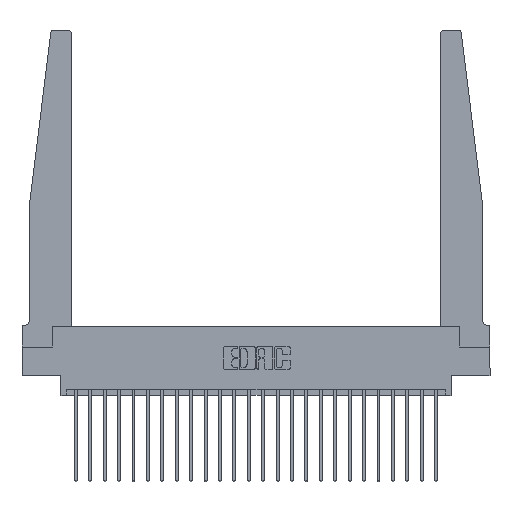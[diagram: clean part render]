
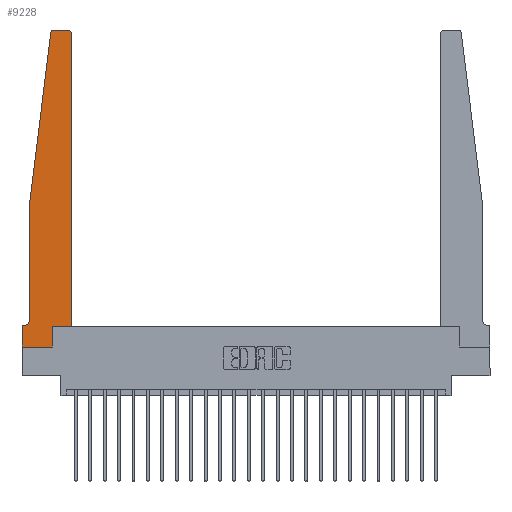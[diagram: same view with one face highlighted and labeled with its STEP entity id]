
A CAD part, top view. The second image highlights one B-rep face of the part: STEP entity #9228.
In plain terms, the highlighted planar face has unit normal (0, 0, 1).
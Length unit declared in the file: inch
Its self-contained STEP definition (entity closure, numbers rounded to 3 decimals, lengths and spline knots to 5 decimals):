
#32 = EDGE_LOOP ( 'NONE', ( #1885, #21672, #7446, #8039, #13606, #23380, #9219, #429, #5406, #1018, #11001, #21397 ) ) ;
#429 = ORIENTED_EDGE ( 'NONE', *, *, #17826, .T. ) ;
#541 = CARTESIAN_POINT ( 'NONE',  ( 0.425, 0.18, 0.37 ) ) ;
#664 = LINE ( 'NONE', #5617, #23602 ) ;
#988 = CARTESIAN_POINT ( 'NONE',  ( 0.065, 0.2375, 0.37 ) ) ;
#1018 = ORIENTED_EDGE ( 'NONE', *, *, #8306, .T. ) ;
#1086 = LINE ( 'NONE', #17839, #20286 ) ;
#1133 = VECTOR ( 'NONE', #13328, 39.37008 ) ;
#1623 = CARTESIAN_POINT ( 'NONE',  ( 0.015, 0.2375, 0.37 ) ) ;
#1766 = CARTESIAN_POINT ( 'NONE',  ( 0.395, 2.72, 0.37 ) ) ;
#1885 = ORIENTED_EDGE ( 'NONE', *, *, #13297, .T. ) ;
#2286 = VECTOR ( 'NONE', #2772, 39.37008 ) ;
#2309 = LINE ( 'NONE', #15104, #1133 ) ;
#2438 = CIRCLE ( 'NONE', #17186, 0.05 ) ;
#2493 = CARTESIAN_POINT ( 'NONE',  ( 0.27653, 2.72, 0.37 ) ) ;
#2772 = DIRECTION ( 'NONE',  ( -1., 0., 0. ) ) ;
#2849 = DIRECTION ( 'NONE',  ( 0., -1., 0. ) ) ;
#3151 = CIRCLE ( 'NONE', #17919, 0.03 ) ;
#3530 = DIRECTION ( 'NONE',  ( -1., 0., 0. ) ) ;
#3667 = LINE ( 'NONE', #15150, #22817 ) ;
#3668 = DIRECTION ( 'NONE',  ( 1., 0., 0. ) ) ;
#4376 = DIRECTION ( 'NONE',  ( 1., 0., 0. ) ) ;
#4550 = DIRECTION ( 'NONE',  ( 1., 0., 0. ) ) ;
#4592 = DIRECTION ( 'NONE',  ( -1., 0., 0. ) ) ;
#4704 = CARTESIAN_POINT ( 'NONE',  ( 0., 0.1875, 0.37 ) ) ;
#4827 = CIRCLE ( 'NONE', #8594, 0.03 ) ;
#5361 = EDGE_CURVE ( 'NONE', #18653, #9847, #21403, .T. ) ;
#5406 = ORIENTED_EDGE ( 'NONE', *, *, #10839, .T. ) ;
#5617 = CARTESIAN_POINT ( 'NONE',  ( 0.425, 0.18, 0.37 ) ) ;
#5650 = CARTESIAN_POINT ( 'NONE',  ( 0.395, 2.75, 0.37 ) ) ;
#6002 = VECTOR ( 'NONE', #2849, 39.37008 ) ;
#6142 = VERTEX_POINT ( 'NONE', #18360 ) ;
#6535 = CARTESIAN_POINT ( 'NONE',  ( 0.065, 1.25, 0.37 ) ) ;
#6582 = DIRECTION ( 'NONE',  ( 0., 0., 1. ) ) ;
#7446 = ORIENTED_EDGE ( 'NONE', *, *, #14765, .T. ) ;
#7843 = LINE ( 'NONE', #12108, #2286 ) ;
#7942 = AXIS2_PLACEMENT_3D ( 'NONE', #4704, #6582, #19578 ) ;
#7964 = VECTOR ( 'NONE', #4550, 39.37008 ) ;
#8039 = ORIENTED_EDGE ( 'NONE', *, *, #5361, .T. ) ;
#8271 = CARTESIAN_POINT ( 'NONE',  ( 0.2605, 0., 0.37 ) ) ;
#8306 = EDGE_CURVE ( 'NONE', #14485, #17707, #2309, .T. ) ;
#8594 = AXIS2_PLACEMENT_3D ( 'NONE', #1766, #14836, #3668 ) ;
#9219 = ORIENTED_EDGE ( 'NONE', *, *, #15057, .T. ) ;
#9228 = ADVANCED_FACE ( 'NONE', ( #13394 ), #21348, .T. ) ;
#9348 = CARTESIAN_POINT ( 'NONE',  ( 0., 0., 0.37 ) ) ;
#9451 = VECTOR ( 'NONE', #4592, 39.37008 ) ;
#9847 = VERTEX_POINT ( 'NONE', #988 ) ;
#10765 = EDGE_CURVE ( 'NONE', #13811, #11398, #4827, .T. ) ;
#10839 = EDGE_CURVE ( 'NONE', #13287, #14485, #3667, .T. ) ;
#11001 = ORIENTED_EDGE ( 'NONE', *, *, #17537, .T. ) ;
#11361 = VECTOR ( 'NONE', #17218, 39.37008 ) ;
#11398 = VERTEX_POINT ( 'NONE', #5650 ) ;
#11630 = CARTESIAN_POINT ( 'NONE',  ( 0.065, 1.25, 0.37 ) ) ;
#11886 = EDGE_CURVE ( 'NONE', #9847, #21925, #2438, .T. ) ;
#12012 = CARTESIAN_POINT ( 'NONE',  ( 0., 0., 0.37 ) ) ;
#12053 = CARTESIAN_POINT ( 'NONE',  ( 0.25, 2.75, 0.37 ) ) ;
#12108 = CARTESIAN_POINT ( 'NONE',  ( 0.065, 0.1875, 0.37 ) ) ;
#13287 = VERTEX_POINT ( 'NONE', #8271 ) ;
#13297 = EDGE_CURVE ( 'NONE', #11398, #17011, #14403, .T. ) ;
#13328 = DIRECTION ( 'NONE',  ( 1., 0., 0. ) ) ;
#13394 = FACE_OUTER_BOUND ( 'NONE', #32, .T. ) ;
#13606 = ORIENTED_EDGE ( 'NONE', *, *, #11886, .T. ) ;
#13811 = VERTEX_POINT ( 'NONE', #21604 ) ;
#14403 = LINE ( 'NONE', #12053, #9451 ) ;
#14485 = VERTEX_POINT ( 'NONE', #19788 ) ;
#14696 = DIRECTION ( 'NONE',  ( 0., 0., -1. ) ) ;
#14765 = EDGE_CURVE ( 'NONE', #6142, #18653, #16291, .T. ) ;
#14836 = DIRECTION ( 'NONE',  ( 0., 0., 1. ) ) ;
#14935 = DIRECTION ( 'NONE',  ( 0., 1., 0. ) ) ;
#15057 = EDGE_CURVE ( 'NONE', #23417, #22206, #1086, .T. ) ;
#15104 = CARTESIAN_POINT ( 'NONE',  ( 0.425, 0.18, 0.37 ) ) ;
#15150 = CARTESIAN_POINT ( 'NONE',  ( 0.2605, 0.18, 0.37 ) ) ;
#15564 = DIRECTION ( 'NONE',  ( 0., 0., 1. ) ) ;
#16291 = LINE ( 'NONE', #11630, #11361 ) ;
#17011 = VERTEX_POINT ( 'NONE', #19065 ) ;
#17015 = DIRECTION ( 'NONE',  ( 0., 1., 0. ) ) ;
#17186 = AXIS2_PLACEMENT_3D ( 'NONE', #1623, #14696, #3530 ) ;
#17218 = DIRECTION ( 'NONE',  ( -0.122, -0.992, 0. ) ) ;
#17452 = CARTESIAN_POINT ( 'NONE',  ( 0.015, 0.1875, 0.37 ) ) ;
#17537 = EDGE_CURVE ( 'NONE', #17707, #13811, #664, .T. ) ;
#17707 = VERTEX_POINT ( 'NONE', #541 ) ;
#17769 = DIRECTION ( 'NONE',  ( 0., -1., 0. ) ) ;
#17826 = EDGE_CURVE ( 'NONE', #22206, #13287, #17858, .T. ) ;
#17839 = CARTESIAN_POINT ( 'NONE',  ( 0., 0., 0.37 ) ) ;
#17858 = LINE ( 'NONE', #12012, #7964 ) ;
#17919 = AXIS2_PLACEMENT_3D ( 'NONE', #2493, #15564, #4376 ) ;
#18356 = CARTESIAN_POINT ( 'NONE',  ( 0., 0.1875, 0.37 ) ) ;
#18360 = CARTESIAN_POINT ( 'NONE',  ( 0.24675, 2.72367, 0.37 ) ) ;
#18653 = VERTEX_POINT ( 'NONE', #22053 ) ;
#19065 = CARTESIAN_POINT ( 'NONE',  ( 0.27653, 2.75, 0.37 ) ) ;
#19578 = DIRECTION ( 'NONE',  ( 1., 0., 0. ) ) ;
#19788 = CARTESIAN_POINT ( 'NONE',  ( 0.2605, 0.18, 0.37 ) ) ;
#20286 = VECTOR ( 'NONE', #17769, 39.37008 ) ;
#20293 = EDGE_CURVE ( 'NONE', #21925, #23417, #7843, .T. ) ;
#20838 = EDGE_CURVE ( 'NONE', #17011, #6142, #3151, .T. ) ;
#21348 = PLANE ( 'NONE',  #7942 ) ;
#21397 = ORIENTED_EDGE ( 'NONE', *, *, #10765, .T. ) ;
#21403 = LINE ( 'NONE', #6535, #6002 ) ;
#21604 = CARTESIAN_POINT ( 'NONE',  ( 0.425, 2.72, 0.37 ) ) ;
#21672 = ORIENTED_EDGE ( 'NONE', *, *, #20838, .T. ) ;
#21925 = VERTEX_POINT ( 'NONE', #17452 ) ;
#22053 = CARTESIAN_POINT ( 'NONE',  ( 0.065, 1.25, 0.37 ) ) ;
#22206 = VERTEX_POINT ( 'NONE', #9348 ) ;
#22817 = VECTOR ( 'NONE', #17015, 39.37008 ) ;
#23380 = ORIENTED_EDGE ( 'NONE', *, *, #20293, .T. ) ;
#23417 = VERTEX_POINT ( 'NONE', #18356 ) ;
#23602 = VECTOR ( 'NONE', #14935, 39.37008 ) ;
